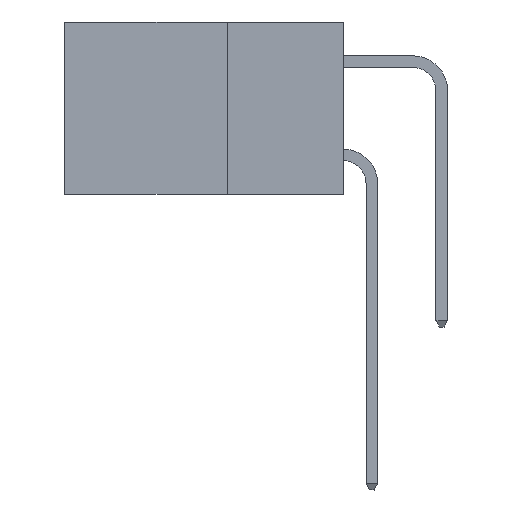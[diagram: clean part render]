
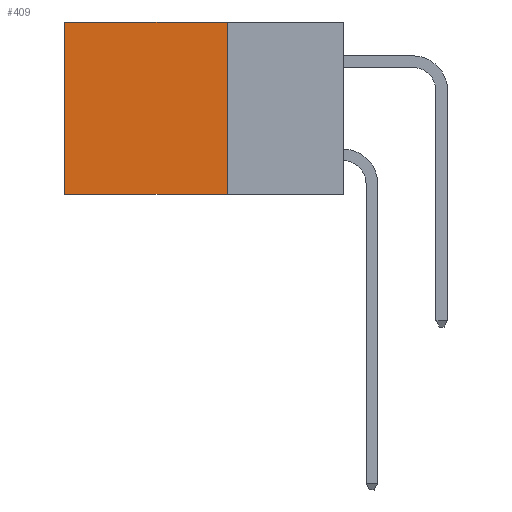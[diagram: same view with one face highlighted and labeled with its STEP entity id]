
A CAD part, left-side view. The second image highlights one B-rep face of the part: STEP entity #409.
In plain terms, the highlighted planar face has unit normal (-1, 0, 0).
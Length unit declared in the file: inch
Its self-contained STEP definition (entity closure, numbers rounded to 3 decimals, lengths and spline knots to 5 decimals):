
#400 = DIRECTION ( 'NONE',  ( 0., 1., 0. ) ) ;
#409 = ADVANCED_FACE ( 'NONE', ( #8541 ), #7313, .F. ) ;
#668 = CARTESIAN_POINT ( 'NONE',  ( 0.2615, 0.6, -0.37 ) ) ;
#827 = DIRECTION ( 'NONE',  ( 0., 0., -1. ) ) ;
#871 = CARTESIAN_POINT ( 'NONE',  ( 0.2615, 0.25, -0.37 ) ) ;
#1590 = ORIENTED_EDGE ( 'NONE', *, *, #6128, .T. ) ;
#1933 = EDGE_CURVE ( 'NONE', #4225, #5028, #6576, .T. ) ;
#1939 = DIRECTION ( 'NONE',  ( 0., 0., -1. ) ) ;
#2090 = LINE ( 'NONE', #871, #13210 ) ;
#2846 = EDGE_CURVE ( 'NONE', #8104, #5028, #12177, .T. ) ;
#2996 = CARTESIAN_POINT ( 'NONE',  ( 0.2615, 0.25, -0.37 ) ) ;
#3068 = EDGE_CURVE ( 'NONE', #6909, #4225, #2090, .T. ) ;
#3259 = VECTOR ( 'NONE', #6983, 39.37008 ) ;
#3627 = DIRECTION ( 'NONE',  ( 0., 1., 0. ) ) ;
#4225 = VERTEX_POINT ( 'NONE', #2996 ) ;
#5028 = VERTEX_POINT ( 'NONE', #668 ) ;
#6128 = EDGE_CURVE ( 'NONE', #6909, #8104, #13273, .T. ) ;
#6576 = LINE ( 'NONE', #15171, #15154 ) ;
#6687 = ORIENTED_EDGE ( 'NONE', *, *, #2846, .T. ) ;
#6909 = VERTEX_POINT ( 'NONE', #14896 ) ;
#6983 = DIRECTION ( 'NONE',  ( 0., 0., -1. ) ) ;
#7313 = PLANE ( 'NONE',  #13301 ) ;
#7884 = VECTOR ( 'NONE', #3627, 39.37008 ) ;
#8104 = VERTEX_POINT ( 'NONE', #10714 ) ;
#8208 = EDGE_LOOP ( 'NONE', ( #6687, #10091, #10076, #1590 ) ) ;
#8541 = FACE_OUTER_BOUND ( 'NONE', #8208, .T. ) ;
#10076 = ORIENTED_EDGE ( 'NONE', *, *, #3068, .F. ) ;
#10091 = ORIENTED_EDGE ( 'NONE', *, *, #1933, .F. ) ;
#10714 = CARTESIAN_POINT ( 'NONE',  ( 0.2615, 0.6, 0. ) ) ;
#12008 = DIRECTION ( 'NONE',  ( 1., 0., 0. ) ) ;
#12177 = LINE ( 'NONE', #13229, #3259 ) ;
#13210 = VECTOR ( 'NONE', #1939, 39.37008 ) ;
#13229 = CARTESIAN_POINT ( 'NONE',  ( 0.2615, 0.6, -0.37 ) ) ;
#13273 = LINE ( 'NONE', #14801, #7884 ) ;
#13301 = AXIS2_PLACEMENT_3D ( 'NONE', #13621, #12008, #827 ) ;
#13621 = CARTESIAN_POINT ( 'NONE',  ( 0.2615, 0.25, -0.37 ) ) ;
#14801 = CARTESIAN_POINT ( 'NONE',  ( 0.2615, 0.25, 0. ) ) ;
#14896 = CARTESIAN_POINT ( 'NONE',  ( 0.2615, 0.25, 0. ) ) ;
#15154 = VECTOR ( 'NONE', #400, 39.37008 ) ;
#15171 = CARTESIAN_POINT ( 'NONE',  ( 0.2615, 0.25, -0.37 ) ) ;
